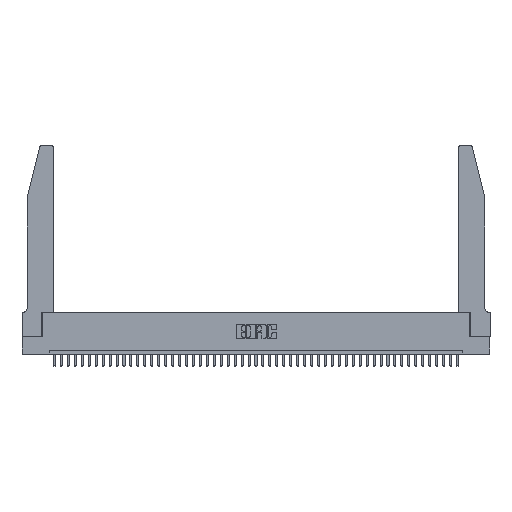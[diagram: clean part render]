
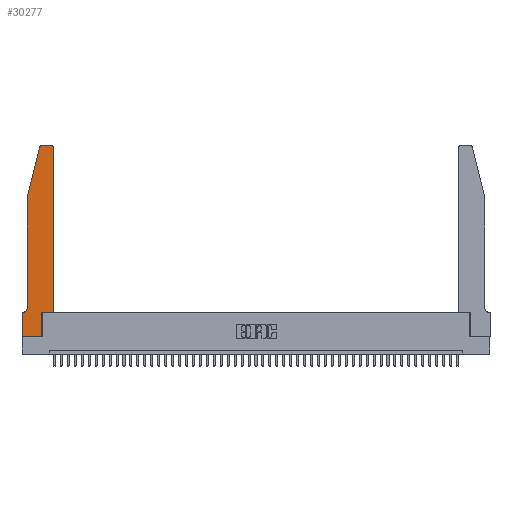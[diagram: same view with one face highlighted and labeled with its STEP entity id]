
A CAD part, top view. The second image highlights one B-rep face of the part: STEP entity #30277.
In plain terms, the highlighted planar face has unit normal (0, 0, 1).
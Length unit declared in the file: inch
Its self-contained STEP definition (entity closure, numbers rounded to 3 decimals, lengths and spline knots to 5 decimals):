
#119 = CARTESIAN_POINT ( 'NONE',  ( 0.0055, 0.35, 0.37 ) ) ;
#532 = VECTOR ( 'NONE', #8831, 39.37008 ) ;
#1003 = ORIENTED_EDGE ( 'NONE', *, *, #22167, .T. ) ;
#1400 = VECTOR ( 'NONE', #23556, 39.37008 ) ;
#1515 = CARTESIAN_POINT ( 'NONE',  ( 0.2865, 0.35, 0.37 ) ) ;
#2769 = LINE ( 'NONE', #37477, #45931 ) ;
#3096 = LINE ( 'NONE', #31685, #42858 ) ;
#3879 = ORIENTED_EDGE ( 'NONE', *, *, #38807, .T. ) ;
#4095 = ORIENTED_EDGE ( 'NONE', *, *, #13045, .T. ) ;
#4732 = DIRECTION ( 'NONE',  ( 0., 0., 1. ) ) ;
#5112 = DIRECTION ( 'NONE',  ( 1., 0., 0. ) ) ;
#5626 = VECTOR ( 'NONE', #34591, 39.37008 ) ;
#6577 = ORIENTED_EDGE ( 'NONE', *, *, #43590, .T. ) ;
#6689 = CARTESIAN_POINT ( 'NONE',  ( 0.284, 2.75, 0.37 ) ) ;
#7096 = VERTEX_POINT ( 'NONE', #14880 ) ;
#7537 = EDGE_CURVE ( 'NONE', #17451, #39460, #2769, .T. ) ;
#8622 = VECTOR ( 'NONE', #17469, 39.37008 ) ;
#8831 = DIRECTION ( 'NONE',  ( 0., 1., 0. ) ) ;
#8869 = VERTEX_POINT ( 'NONE', #41221 ) ;
#8970 = AXIS2_PLACEMENT_3D ( 'NONE', #37897, #4732, #44887 ) ;
#9998 = DIRECTION ( 'NONE',  ( 0., 0., -1. ) ) ;
#10127 = DIRECTION ( 'NONE',  ( 0., 0., 1. ) ) ;
#10265 = AXIS2_PLACEMENT_3D ( 'NONE', #13080, #20383, #45626 ) ;
#11601 = VECTOR ( 'NONE', #25697, 39.37008 ) ;
#11611 = VERTEX_POINT ( 'NONE', #38706 ) ;
#12577 = CARTESIAN_POINT ( 'NONE',  ( 0.4505, 2.72, 0.37 ) ) ;
#12591 = CARTESIAN_POINT ( 'NONE',  ( 0.25487, 2.72718, 0.37 ) ) ;
#12714 = AXIS2_PLACEMENT_3D ( 'NONE', #27594, #9998, #31427 ) ;
#12889 = VERTEX_POINT ( 'NONE', #27737 ) ;
#13045 = EDGE_CURVE ( 'NONE', #11611, #31659, #18798, .T. ) ;
#13080 = CARTESIAN_POINT ( 'NONE',  ( 0.284, 2.72, 0.37 ) ) ;
#13344 = LINE ( 'NONE', #36252, #11601 ) ;
#14880 = CARTESIAN_POINT ( 'NONE',  ( 0.2865, 0., 0.37 ) ) ;
#15693 = DIRECTION ( 'NONE',  ( 0., 1., 0. ) ) ;
#15981 = LINE ( 'NONE', #32129, #8622 ) ;
#17451 = VERTEX_POINT ( 'NONE', #23338 ) ;
#17469 = DIRECTION ( 'NONE',  ( -1., 0., 0. ) ) ;
#17479 = CARTESIAN_POINT ( 'NONE',  ( 0., 0., 0.37 ) ) ;
#17618 = ORIENTED_EDGE ( 'NONE', *, *, #40680, .T. ) ;
#18734 = VERTEX_POINT ( 'NONE', #30725 ) ;
#18798 = LINE ( 'NONE', #17479, #30208 ) ;
#18882 = ORIENTED_EDGE ( 'NONE', *, *, #7537, .T. ) ;
#20103 = CARTESIAN_POINT ( 'NONE',  ( 0.0755, 2., 0.37 ) ) ;
#20228 = VERTEX_POINT ( 'NONE', #12591 ) ;
#20383 = DIRECTION ( 'NONE',  ( 0., 0., 1. ) ) ;
#20412 = ORIENTED_EDGE ( 'NONE', *, *, #32241, .T. ) ;
#21985 = EDGE_CURVE ( 'NONE', #8869, #17451, #37975, .T. ) ;
#22054 = EDGE_CURVE ( 'NONE', #39460, #12889, #46549, .T. ) ;
#22167 = EDGE_CURVE ( 'NONE', #32927, #20228, #40249, .T. ) ;
#22545 = CIRCLE ( 'NONE', #12714, 0.07 ) ;
#23282 = EDGE_LOOP ( 'NONE', ( #39479, #1003, #6577, #20412, #17618, #28958, #4095, #44854, #3879, #31552, #18882, #44603 ) ) ;
#23338 = CARTESIAN_POINT ( 'NONE',  ( 0.4505, 0.35, 0.37 ) ) ;
#23552 = VERTEX_POINT ( 'NONE', #20103 ) ;
#23556 = DIRECTION ( 'NONE',  ( -0.239, -0.971, 0. ) ) ;
#25697 = DIRECTION ( 'NONE',  ( 1., 0., 0. ) ) ;
#26449 = PLANE ( 'NONE',  #8970 ) ;
#27594 = CARTESIAN_POINT ( 'NONE',  ( 0.0055, 0.42, 0.37 ) ) ;
#27737 = CARTESIAN_POINT ( 'NONE',  ( 0.4205, 2.75, 0.37 ) ) ;
#28410 = VECTOR ( 'NONE', #40752, 39.37008 ) ;
#28661 = DIRECTION ( 'NONE',  ( 0., -1., 0. ) ) ;
#28823 = FACE_OUTER_BOUND ( 'NONE', #23282, .T. ) ;
#28958 = ORIENTED_EDGE ( 'NONE', *, *, #40603, .T. ) ;
#30208 = VECTOR ( 'NONE', #39695, 39.37008 ) ;
#30277 = ADVANCED_FACE ( 'NONE', ( #28823 ), #26449, .T. ) ;
#30725 = CARTESIAN_POINT ( 'NONE',  ( 0.0755, 0.42, 0.37 ) ) ;
#31427 = DIRECTION ( 'NONE',  ( -1., 0., 0. ) ) ;
#31552 = ORIENTED_EDGE ( 'NONE', *, *, #21985, .T. ) ;
#31659 = VERTEX_POINT ( 'NONE', #44045 ) ;
#31685 = CARTESIAN_POINT ( 'NONE',  ( 0.0755, 2., 0.37 ) ) ;
#32129 = CARTESIAN_POINT ( 'NONE',  ( 0.2605, 2.75, 0.37 ) ) ;
#32241 = EDGE_CURVE ( 'NONE', #23552, #18734, #3096, .T. ) ;
#32744 = LINE ( 'NONE', #34730, #1400 ) ;
#32927 = VERTEX_POINT ( 'NONE', #6689 ) ;
#34448 = CARTESIAN_POINT ( 'NONE',  ( 0.0755, 0.35, 0.37 ) ) ;
#34591 = DIRECTION ( 'NONE',  ( -1., 0., 0. ) ) ;
#34730 = CARTESIAN_POINT ( 'NONE',  ( 0.0755, 2., 0.37 ) ) ;
#36252 = CARTESIAN_POINT ( 'NONE',  ( 0., 0., 0.37 ) ) ;
#37267 = CARTESIAN_POINT ( 'NONE',  ( 0.4505, 0.35, 0.37 ) ) ;
#37313 = CARTESIAN_POINT ( 'NONE',  ( 0.4205, 2.72, 0.37 ) ) ;
#37477 = CARTESIAN_POINT ( 'NONE',  ( 0.4505, 0.35, 0.37 ) ) ;
#37897 = CARTESIAN_POINT ( 'NONE',  ( 0., 0.35, 0.37 ) ) ;
#37975 = LINE ( 'NONE', #37267, #28410 ) ;
#38706 = CARTESIAN_POINT ( 'NONE',  ( 0., 0.35, 0.37 ) ) ;
#38807 = EDGE_CURVE ( 'NONE', #7096, #8869, #42077, .T. ) ;
#39220 = VERTEX_POINT ( 'NONE', #119 ) ;
#39460 = VERTEX_POINT ( 'NONE', #12577 ) ;
#39479 = ORIENTED_EDGE ( 'NONE', *, *, #45826, .T. ) ;
#39695 = DIRECTION ( 'NONE',  ( 0., -1., 0. ) ) ;
#40249 = CIRCLE ( 'NONE', #10265, 0.03 ) ;
#40603 = EDGE_CURVE ( 'NONE', #39220, #11611, #42570, .T. ) ;
#40680 = EDGE_CURVE ( 'NONE', #18734, #39220, #22545, .T. ) ;
#40752 = DIRECTION ( 'NONE',  ( 1., 0., 0. ) ) ;
#40904 = AXIS2_PLACEMENT_3D ( 'NONE', #37313, #10127, #5112 ) ;
#41221 = CARTESIAN_POINT ( 'NONE',  ( 0.2865, 0.35, 0.37 ) ) ;
#42077 = LINE ( 'NONE', #1515, #532 ) ;
#42570 = LINE ( 'NONE', #34448, #5626 ) ;
#42858 = VECTOR ( 'NONE', #28661, 39.37008 ) ;
#43590 = EDGE_CURVE ( 'NONE', #20228, #23552, #32744, .T. ) ;
#43826 = EDGE_CURVE ( 'NONE', #31659, #7096, #13344, .T. ) ;
#44045 = CARTESIAN_POINT ( 'NONE',  ( 0., 0., 0.37 ) ) ;
#44603 = ORIENTED_EDGE ( 'NONE', *, *, #22054, .T. ) ;
#44854 = ORIENTED_EDGE ( 'NONE', *, *, #43826, .T. ) ;
#44887 = DIRECTION ( 'NONE',  ( 1., 0., 0. ) ) ;
#45626 = DIRECTION ( 'NONE',  ( 1., 0., 0. ) ) ;
#45826 = EDGE_CURVE ( 'NONE', #12889, #32927, #15981, .T. ) ;
#45931 = VECTOR ( 'NONE', #15693, 39.37008 ) ;
#46549 = CIRCLE ( 'NONE', #40904, 0.03 ) ;
